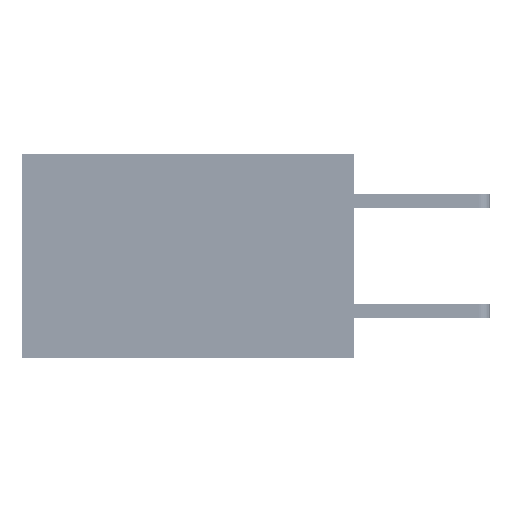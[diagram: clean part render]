
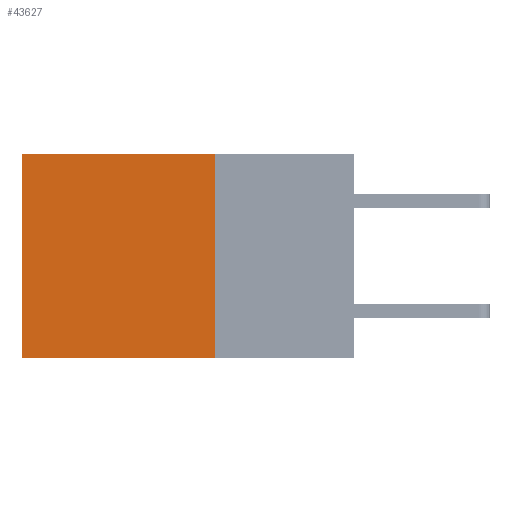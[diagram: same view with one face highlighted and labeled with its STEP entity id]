
A CAD part, left-side view. The second image highlights one B-rep face of the part: STEP entity #43627.
In plain terms, the highlighted planar face has unit normal (-1, 0, 0).
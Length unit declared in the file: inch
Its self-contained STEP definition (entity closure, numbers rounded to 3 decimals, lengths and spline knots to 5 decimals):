
#503 = CARTESIAN_POINT ( 'NONE',  ( 0.2875, 0.25, 0. ) ) ;
#827 = DIRECTION ( 'NONE',  ( 0., 0., -1. ) ) ;
#3022 = VECTOR ( 'NONE', #33702, 39.37008 ) ;
#3613 = CARTESIAN_POINT ( 'NONE',  ( 0.2875, 0.6, 0. ) ) ;
#7191 = ORIENTED_EDGE ( 'NONE', *, *, #33863, .F. ) ;
#7470 = CARTESIAN_POINT ( 'NONE',  ( 0.2875, 0.25, 0. ) ) ;
#7699 = VERTEX_POINT ( 'NONE', #38879 ) ;
#8248 = CARTESIAN_POINT ( 'NONE',  ( 0.2875, 0.25, -0.37 ) ) ;
#8470 = CARTESIAN_POINT ( 'NONE',  ( 0.2875, 0.6, 0. ) ) ;
#9080 = CARTESIAN_POINT ( 'NONE',  ( 0.2875, 0.25, 0. ) ) ;
#10702 = ORIENTED_EDGE ( 'NONE', *, *, #42895, .F. ) ;
#12116 = CARTESIAN_POINT ( 'NONE',  ( 0.2875, 0.25, -0.37 ) ) ;
#13117 = VECTOR ( 'NONE', #34334, 39.37008 ) ;
#13574 = EDGE_CURVE ( 'NONE', #33163, #7699, #35502, .T. ) ;
#15727 = ORIENTED_EDGE ( 'NONE', *, *, #13574, .T. ) ;
#20958 = ORIENTED_EDGE ( 'NONE', *, *, #23833, .T. ) ;
#23523 = LINE ( 'NONE', #9080, #32275 ) ;
#23833 = EDGE_CURVE ( 'NONE', #30145, #33163, #23523, .T. ) ;
#24732 = FACE_OUTER_BOUND ( 'NONE', #40923, .T. ) ;
#26782 = DIRECTION ( 'NONE',  ( 1., 0., 0. ) ) ;
#29338 = VERTEX_POINT ( 'NONE', #12116 ) ;
#30145 = VERTEX_POINT ( 'NONE', #35455 ) ;
#32275 = VECTOR ( 'NONE', #32530, 39.37008 ) ;
#32530 = DIRECTION ( 'NONE',  ( 0., 1., 0. ) ) ;
#33163 = VERTEX_POINT ( 'NONE', #8470 ) ;
#33702 = DIRECTION ( 'NONE',  ( 0., 0., -1. ) ) ;
#33863 = EDGE_CURVE ( 'NONE', #29338, #7699, #34775, .T. ) ;
#34334 = DIRECTION ( 'NONE',  ( 0., 1., 0. ) ) ;
#34336 = VECTOR ( 'NONE', #37198, 39.37008 ) ;
#34775 = LINE ( 'NONE', #8248, #13117 ) ;
#35455 = CARTESIAN_POINT ( 'NONE',  ( 0.2875, 0.25, 0. ) ) ;
#35502 = LINE ( 'NONE', #3613, #34336 ) ;
#35875 = LINE ( 'NONE', #7470, #3022 ) ;
#37198 = DIRECTION ( 'NONE',  ( 0., 0., -1. ) ) ;
#38879 = CARTESIAN_POINT ( 'NONE',  ( 0.2875, 0.6, -0.37 ) ) ;
#40831 = PLANE ( 'NONE',  #43407 ) ;
#40923 = EDGE_LOOP ( 'NONE', ( #15727, #7191, #10702, #20958 ) ) ;
#42895 = EDGE_CURVE ( 'NONE', #30145, #29338, #35875, .T. ) ;
#43407 = AXIS2_PLACEMENT_3D ( 'NONE', #503, #26782, #827 ) ;
#43627 = ADVANCED_FACE ( 'NONE', ( #24732 ), #40831, .F. ) ;
